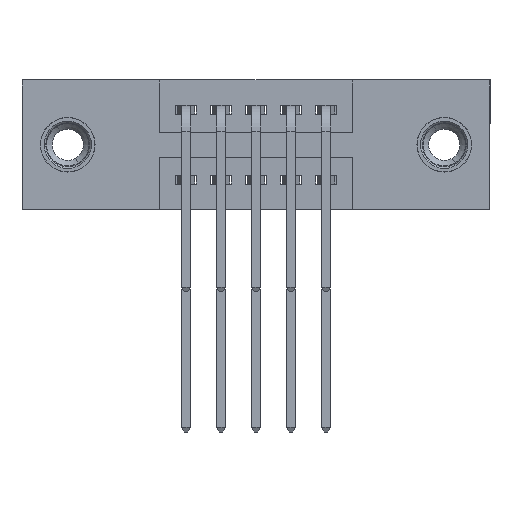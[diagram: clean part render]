
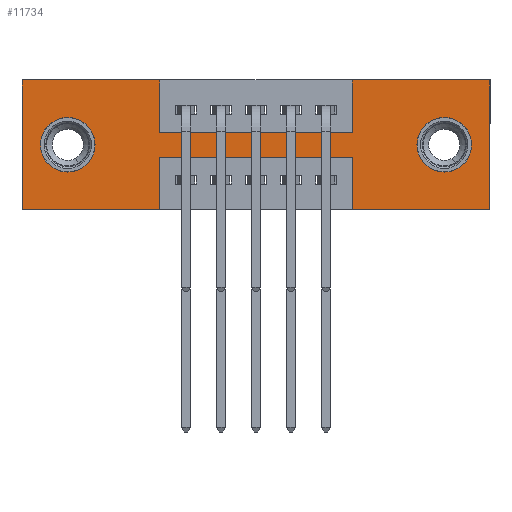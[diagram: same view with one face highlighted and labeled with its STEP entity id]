
A CAD part, front view. The second image highlights one B-rep face of the part: STEP entity #11734.
In plain terms, the highlighted planar face has unit normal (0, -1, 0).
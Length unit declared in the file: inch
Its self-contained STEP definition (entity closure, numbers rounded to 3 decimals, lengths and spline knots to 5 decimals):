
#31 = CARTESIAN_POINT ( 'NONE',  ( 1.205, 0., -0.107 ) ) ;
#228 = DIRECTION ( 'NONE',  ( 0., 1., 0. ) ) ;
#250 = CARTESIAN_POINT ( 'NONE',  ( 0.3925, 0., 0. ) ) ;
#251 = DIRECTION ( 'NONE',  ( 0., 0., 1. ) ) ;
#370 = ORIENTED_EDGE ( 'NONE', *, *, #1167, .F. ) ;
#480 = CARTESIAN_POINT ( 'NONE',  ( 0.13, 0., -0.263 ) ) ;
#545 = VERTEX_POINT ( 'NONE', #5336 ) ;
#587 = EDGE_CURVE ( 'NONE', #13078, #5229, #7778, .T. ) ;
#627 = CARTESIAN_POINT ( 'NONE',  ( 0., 0., -0.37 ) ) ;
#908 = VERTEX_POINT ( 'NONE', #12080 ) ;
#917 = EDGE_CURVE ( 'NONE', #2042, #15052, #5031, .T. ) ;
#1053 = EDGE_LOOP ( 'NONE', ( #11016, #6859 ) ) ;
#1148 = VERTEX_POINT ( 'NONE', #9691 ) ;
#1167 = EDGE_CURVE ( 'NONE', #8975, #908, #15055, .T. ) ;
#1413 = FACE_BOUND ( 'NONE', #1053, .T. ) ;
#1471 = DIRECTION ( 'NONE',  ( 0., 0., 1. ) ) ;
#1521 = DIRECTION ( 'NONE',  ( 0., 0., -1. ) ) ;
#1544 = EDGE_CURVE ( 'NONE', #14268, #13135, #4845, .T. ) ;
#1915 = VECTOR ( 'NONE', #13685, 39.37008 ) ;
#2042 = VERTEX_POINT ( 'NONE', #8870 ) ;
#2249 = EDGE_LOOP ( 'NONE', ( #3758, #7407 ) ) ;
#2383 = AXIS2_PLACEMENT_3D ( 'NONE', #9144, #9757, #7325 ) ;
#2607 = CARTESIAN_POINT ( 'NONE',  ( 0.3925, 0., 0. ) ) ;
#2659 = LINE ( 'NONE', #3700, #8167 ) ;
#3053 = CARTESIAN_POINT ( 'NONE',  ( 0., 0., -0.37 ) ) ;
#3060 = EDGE_LOOP ( 'NONE', ( #5351, #370, #8881, #6985, #7296, #6162, #9497, #11077, #9698, #13550, #8195, #11442 ) ) ;
#3218 = LINE ( 'NONE', #14260, #5756 ) ;
#3578 = LINE ( 'NONE', #8592, #12446 ) ;
#3689 = EDGE_CURVE ( 'NONE', #13135, #8975, #13331, .T. ) ;
#3700 = CARTESIAN_POINT ( 'NONE',  ( 0., 0., 0. ) ) ;
#3758 = ORIENTED_EDGE ( 'NONE', *, *, #7676, .T. ) ;
#3994 = VERTEX_POINT ( 'NONE', #31 ) ;
#4105 = VECTOR ( 'NONE', #5487, 39.37008 ) ;
#4267 = CARTESIAN_POINT ( 'NONE',  ( 0., 0., -0.37 ) ) ;
#4420 = EDGE_CURVE ( 'NONE', #14964, #545, #4768, .T. ) ;
#4683 = CARTESIAN_POINT ( 'NONE',  ( 0., 0., 0. ) ) ;
#4768 = LINE ( 'NONE', #4683, #13321 ) ;
#4789 = CARTESIAN_POINT ( 'NONE',  ( 1.335, 0., -0.37 ) ) ;
#4845 = LINE ( 'NONE', #6475, #6131 ) ;
#4850 = CARTESIAN_POINT ( 'NONE',  ( 0.3925, 0., -0.22 ) ) ;
#5031 = CIRCLE ( 'NONE', #13877, 0.078 ) ;
#5229 = VERTEX_POINT ( 'NONE', #3053 ) ;
#5251 = LINE ( 'NONE', #9275, #8769 ) ;
#5336 = CARTESIAN_POINT ( 'NONE',  ( 1.335, 0., 0. ) ) ;
#5351 = ORIENTED_EDGE ( 'NONE', *, *, #13756, .F. ) ;
#5487 = DIRECTION ( 'NONE',  ( -1., 0., 0. ) ) ;
#5501 = EDGE_CURVE ( 'NONE', #13577, #13003, #15125, .T. ) ;
#5756 = VECTOR ( 'NONE', #8211, 39.37008 ) ;
#5811 = CARTESIAN_POINT ( 'NONE',  ( 0.9425, 0., -0.22 ) ) ;
#5832 = DIRECTION ( 'NONE',  ( 0., 1., 0. ) ) ;
#5940 = DIRECTION ( 'NONE',  ( 0., 0., 1. ) ) ;
#6109 = DIRECTION ( 'NONE',  ( 1., 0., 0. ) ) ;
#6131 = VECTOR ( 'NONE', #8955, 39.37008 ) ;
#6162 = ORIENTED_EDGE ( 'NONE', *, *, #4420, .F. ) ;
#6164 = EDGE_CURVE ( 'NONE', #13003, #14964, #5251, .T. ) ;
#6473 = DIRECTION ( 'NONE',  ( 0., -1., 0. ) ) ;
#6475 = CARTESIAN_POINT ( 'NONE',  ( 0., 0., -0.37 ) ) ;
#6654 = EDGE_CURVE ( 'NONE', #1148, #3994, #8392, .T. ) ;
#6859 = ORIENTED_EDGE ( 'NONE', *, *, #8994, .T. ) ;
#6985 = ORIENTED_EDGE ( 'NONE', *, *, #1544, .F. ) ;
#7278 = DIRECTION ( 'NONE',  ( 1., 0., 0. ) ) ;
#7296 = ORIENTED_EDGE ( 'NONE', *, *, #13676, .F. ) ;
#7325 = DIRECTION ( 'NONE',  ( 0., 0., -1. ) ) ;
#7407 = ORIENTED_EDGE ( 'NONE', *, *, #6654, .T. ) ;
#7547 = VECTOR ( 'NONE', #5940, 39.37008 ) ;
#7666 = PLANE ( 'NONE',  #9611 ) ;
#7676 = EDGE_CURVE ( 'NONE', #3994, #1148, #13574, .T. ) ;
#7778 = LINE ( 'NONE', #4267, #4105 ) ;
#8002 = VECTOR ( 'NONE', #1521, 39.37008 ) ;
#8075 = CARTESIAN_POINT ( 'NONE',  ( 0.9425, 0., -0.37 ) ) ;
#8095 = EDGE_CURVE ( 'NONE', #12885, #8494, #3578, .T. ) ;
#8167 = VECTOR ( 'NONE', #1471, 39.37008 ) ;
#8179 = LINE ( 'NONE', #250, #1915 ) ;
#8195 = ORIENTED_EDGE ( 'NONE', *, *, #13731, .F. ) ;
#8211 = DIRECTION ( 'NONE',  ( 0., 0., -1. ) ) ;
#8392 = CIRCLE ( 'NONE', #15326, 0.078 ) ;
#8494 = VERTEX_POINT ( 'NONE', #2607 ) ;
#8592 = CARTESIAN_POINT ( 'NONE',  ( 0., 0., 0. ) ) ;
#8633 = DIRECTION ( 'NONE',  ( 0., 1., 0. ) ) ;
#8769 = VECTOR ( 'NONE', #12726, 39.37008 ) ;
#8870 = CARTESIAN_POINT ( 'NONE',  ( 0.13, 0., -0.107 ) ) ;
#8881 = ORIENTED_EDGE ( 'NONE', *, *, #3689, .F. ) ;
#8939 = CARTESIAN_POINT ( 'NONE',  ( 0.9425, 0., -0.15 ) ) ;
#8955 = DIRECTION ( 'NONE',  ( -1., 0., 0. ) ) ;
#8975 = VERTEX_POINT ( 'NONE', #5811 ) ;
#8994 = EDGE_CURVE ( 'NONE', #15052, #2042, #14667, .T. ) ;
#9144 = CARTESIAN_POINT ( 'NONE',  ( 1.205, 0., -0.185 ) ) ;
#9152 = CARTESIAN_POINT ( 'NONE',  ( 0.3925, 0., -0.37 ) ) ;
#9275 = CARTESIAN_POINT ( 'NONE',  ( 0.9425, 0., 0. ) ) ;
#9310 = CARTESIAN_POINT ( 'NONE',  ( 1.205, 0., -0.185 ) ) ;
#9318 = DIRECTION ( 'NONE',  ( 1., 0., 0. ) ) ;
#9497 = ORIENTED_EDGE ( 'NONE', *, *, #6164, .F. ) ;
#9545 = CARTESIAN_POINT ( 'NONE',  ( 0.3925, 0., -0.37 ) ) ;
#9611 = AXIS2_PLACEMENT_3D ( 'NONE', #627, #6473, #13741 ) ;
#9644 = CARTESIAN_POINT ( 'NONE',  ( 0.9425, 0., 0. ) ) ;
#9691 = CARTESIAN_POINT ( 'NONE',  ( 1.205, 0., -0.263 ) ) ;
#9698 = ORIENTED_EDGE ( 'NONE', *, *, #13386, .F. ) ;
#9757 = DIRECTION ( 'NONE',  ( 0., 1., 0. ) ) ;
#10766 = AXIS2_PLACEMENT_3D ( 'NONE', #13784, #228, #11886 ) ;
#10814 = FACE_BOUND ( 'NONE', #2249, .T. ) ;
#10896 = CARTESIAN_POINT ( 'NONE',  ( 0.3925, 0., -0.15 ) ) ;
#10963 = CARTESIAN_POINT ( 'NONE',  ( 0.13, 0., -0.185 ) ) ;
#11016 = ORIENTED_EDGE ( 'NONE', *, *, #917, .T. ) ;
#11077 = ORIENTED_EDGE ( 'NONE', *, *, #5501, .F. ) ;
#11442 = ORIENTED_EDGE ( 'NONE', *, *, #587, .F. ) ;
#11597 = DIRECTION ( 'NONE',  ( 0., 0., -1. ) ) ;
#11734 = ADVANCED_FACE ( 'NONE', ( #10814, #1413, #13270 ), #7666, .T. ) ;
#11886 = DIRECTION ( 'NONE',  ( 0., 0., 1. ) ) ;
#11899 = VECTOR ( 'NONE', #12060, 39.37008 ) ;
#12060 = DIRECTION ( 'NONE',  ( -1., 0., 0. ) ) ;
#12080 = CARTESIAN_POINT ( 'NONE',  ( 0.3925, 0., -0.22 ) ) ;
#12446 = VECTOR ( 'NONE', #6109, 39.37008 ) ;
#12726 = DIRECTION ( 'NONE',  ( 0., 0., 1. ) ) ;
#12885 = VERTEX_POINT ( 'NONE', #13443 ) ;
#13003 = VERTEX_POINT ( 'NONE', #8939 ) ;
#13078 = VERTEX_POINT ( 'NONE', #9152 ) ;
#13135 = VERTEX_POINT ( 'NONE', #15036 ) ;
#13270 = FACE_OUTER_BOUND ( 'NONE', #3060, .T. ) ;
#13321 = VECTOR ( 'NONE', #9318, 39.37008 ) ;
#13331 = LINE ( 'NONE', #8075, #7547 ) ;
#13386 = EDGE_CURVE ( 'NONE', #8494, #13577, #8179, .T. ) ;
#13443 = CARTESIAN_POINT ( 'NONE',  ( 0., 0., 0. ) ) ;
#13458 = VECTOR ( 'NONE', #7278, 39.37008 ) ;
#13550 = ORIENTED_EDGE ( 'NONE', *, *, #8095, .F. ) ;
#13569 = LINE ( 'NONE', #9545, #8002 ) ;
#13574 = CIRCLE ( 'NONE', #2383, 0.078 ) ;
#13577 = VERTEX_POINT ( 'NONE', #13943 ) ;
#13676 = EDGE_CURVE ( 'NONE', #545, #14268, #3218, .T. ) ;
#13685 = DIRECTION ( 'NONE',  ( 0., 0., -1. ) ) ;
#13731 = EDGE_CURVE ( 'NONE', #5229, #12885, #2659, .T. ) ;
#13741 = DIRECTION ( 'NONE',  ( 0., 0., -1. ) ) ;
#13756 = EDGE_CURVE ( 'NONE', #908, #13078, #13569, .T. ) ;
#13784 = CARTESIAN_POINT ( 'NONE',  ( 0.13, 0., -0.185 ) ) ;
#13877 = AXIS2_PLACEMENT_3D ( 'NONE', #10963, #8633, #251 ) ;
#13943 = CARTESIAN_POINT ( 'NONE',  ( 0.3925, 0., -0.15 ) ) ;
#14260 = CARTESIAN_POINT ( 'NONE',  ( 1.335, 0., 0. ) ) ;
#14268 = VERTEX_POINT ( 'NONE', #4789 ) ;
#14667 = CIRCLE ( 'NONE', #10766, 0.078 ) ;
#14964 = VERTEX_POINT ( 'NONE', #9644 ) ;
#15036 = CARTESIAN_POINT ( 'NONE',  ( 0.9425, 0., -0.37 ) ) ;
#15052 = VERTEX_POINT ( 'NONE', #480 ) ;
#15055 = LINE ( 'NONE', #4850, #11899 ) ;
#15125 = LINE ( 'NONE', #10896, #13458 ) ;
#15326 = AXIS2_PLACEMENT_3D ( 'NONE', #9310, #5832, #11597 ) ;
